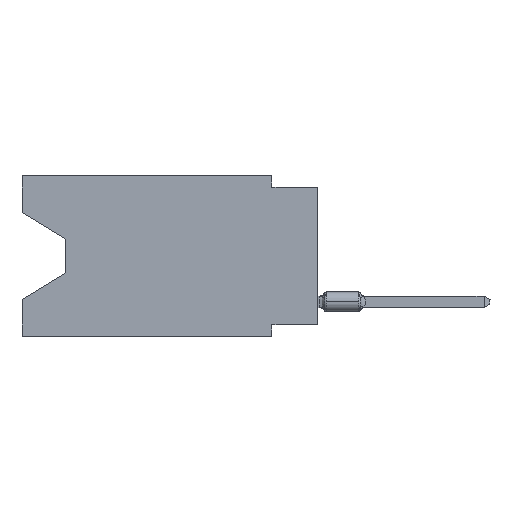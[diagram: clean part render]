
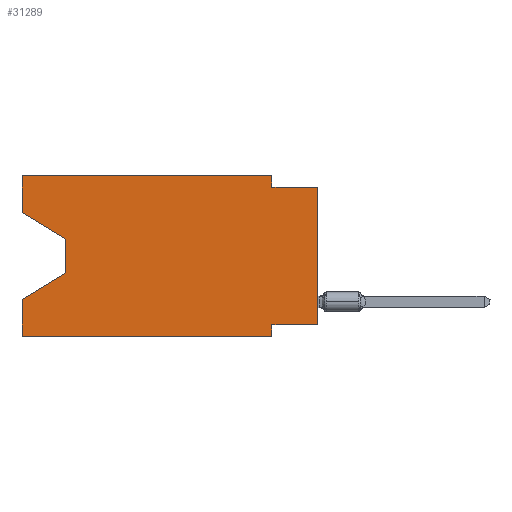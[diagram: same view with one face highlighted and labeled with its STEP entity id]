
A CAD part, left-side view. The second image highlights one B-rep face of the part: STEP entity #31289.
In plain terms, the highlighted planar face has unit normal (-1, 0, 0).
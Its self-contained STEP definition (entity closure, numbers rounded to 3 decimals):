
#288 = VERTEX_POINT ( 'NONE', #8696 ) ;
#362 = LINE ( 'NONE', #21409, #45308 ) ;
#1488 = CARTESIAN_POINT ( 'NONE',  ( 0., 13.97, -3.505 ) ) ;
#1493 = CARTESIAN_POINT ( 'NONE',  ( 0., 16.383, 0. ) ) ;
#2668 = VERTEX_POINT ( 'NONE', #25095 ) ;
#2764 = VECTOR ( 'NONE', #37496, 1000. ) ;
#3194 = ORIENTED_EDGE ( 'NONE', *, *, #24355, .F. ) ;
#3503 = ORIENTED_EDGE ( 'NONE', *, *, #11432, .T. ) ;
#3954 = VECTOR ( 'NONE', #22045, 1000. ) ;
#4253 = DIRECTION ( 'NONE',  ( 0., 1., 0. ) ) ;
#5149 = CARTESIAN_POINT ( 'NONE',  ( 0., 13.97, -5.385 ) ) ;
#5156 = EDGE_CURVE ( 'NONE', #2668, #15864, #10534, .T. ) ;
#5335 = CARTESIAN_POINT ( 'NONE',  ( 0., 16.383, -8.89 ) ) ;
#5417 = VERTEX_POINT ( 'NONE', #44933 ) ;
#5556 = VERTEX_POINT ( 'NONE', #24433 ) ;
#6807 = EDGE_CURVE ( 'NONE', #31838, #288, #43417, .T. ) ;
#7279 = CARTESIAN_POINT ( 'NONE',  ( 0., 16.383, 0. ) ) ;
#7749 = VECTOR ( 'NONE', #23061, 1000. ) ;
#8260 = CARTESIAN_POINT ( 'NONE',  ( 0., 16.383, -6.852 ) ) ;
#8550 = ORIENTED_EDGE ( 'NONE', *, *, #21426, .T. ) ;
#8588 = LINE ( 'NONE', #1493, #9632 ) ;
#8696 = CARTESIAN_POINT ( 'NONE',  ( 0., 2.54, -8.255 ) ) ;
#9279 = DIRECTION ( 'NONE',  ( 0., 0., -1. ) ) ;
#9632 = VECTOR ( 'NONE', #38292, 1000. ) ;
#9767 = VECTOR ( 'NONE', #20304, 1000. ) ;
#10534 = LINE ( 'NONE', #21626, #24575 ) ;
#11329 = LINE ( 'NONE', #5149, #2764 ) ;
#11432 = EDGE_CURVE ( 'NONE', #31838, #26762, #362, .T. ) ;
#11551 = DIRECTION ( 'NONE',  ( 0., 0., 1. ) ) ;
#12042 = ORIENTED_EDGE ( 'NONE', *, *, #6807, .F. ) ;
#13293 = VERTEX_POINT ( 'NONE', #8260 ) ;
#14489 = CARTESIAN_POINT ( 'NONE',  ( 0., 16.383, -2.038 ) ) ;
#15470 = EDGE_CURVE ( 'NONE', #21038, #5556, #22848, .T. ) ;
#15864 = VERTEX_POINT ( 'NONE', #22562 ) ;
#16681 = ORIENTED_EDGE ( 'NONE', *, *, #34973, .T. ) ;
#17640 = DIRECTION ( 'NONE',  ( 0., 0., -1. ) ) ;
#18025 = VECTOR ( 'NONE', #45277, 1000. ) ;
#18205 = EDGE_LOOP ( 'NONE', ( #16681, #8550, #35787, #31002, #39448, #19324, #12042, #3503, #3194, #38494, #41370, #25934 ) ) ;
#18444 = CARTESIAN_POINT ( 'NONE',  ( 0., 0., -8.255 ) ) ;
#18653 = EDGE_CURVE ( 'NONE', #22435, #13293, #11329, .T. ) ;
#19324 = ORIENTED_EDGE ( 'NONE', *, *, #32594, .F. ) ;
#19439 = VECTOR ( 'NONE', #9279, 1000. ) ;
#20145 = VECTOR ( 'NONE', #4253, 1000. ) ;
#20213 = VERTEX_POINT ( 'NONE', #24103 ) ;
#20304 = DIRECTION ( 'NONE',  ( 0., -1., 0. ) ) ;
#21038 = VERTEX_POINT ( 'NONE', #41430 ) ;
#21409 = CARTESIAN_POINT ( 'NONE',  ( 0., 0., 0. ) ) ;
#21426 = EDGE_CURVE ( 'NONE', #5417, #22435, #44442, .T. ) ;
#21626 = CARTESIAN_POINT ( 'NONE',  ( 0., 2.54, 0. ) ) ;
#22045 = DIRECTION ( 'NONE',  ( 0., -1., 0. ) ) ;
#22176 = CARTESIAN_POINT ( 'NONE',  ( 0., 16.383, 0. ) ) ;
#22183 = FACE_OUTER_BOUND ( 'NONE', #18205, .T. ) ;
#22435 = VERTEX_POINT ( 'NONE', #28856 ) ;
#22562 = CARTESIAN_POINT ( 'NONE',  ( 0., 2.54, -0.635 ) ) ;
#22848 = LINE ( 'NONE', #5335, #7749 ) ;
#23061 = DIRECTION ( 'NONE',  ( 0., -1., 0. ) ) ;
#24103 = CARTESIAN_POINT ( 'NONE',  ( 0., 16.383, 0. ) ) ;
#24355 = EDGE_CURVE ( 'NONE', #15864, #26762, #34714, .T. ) ;
#24433 = CARTESIAN_POINT ( 'NONE',  ( 0., 2.54, -8.89 ) ) ;
#24575 = VECTOR ( 'NONE', #17640, 1000. ) ;
#25095 = CARTESIAN_POINT ( 'NONE',  ( 0., 2.54, 0. ) ) ;
#25823 = LINE ( 'NONE', #14489, #29602 ) ;
#25934 = ORIENTED_EDGE ( 'NONE', *, *, #32847, .F. ) ;
#26762 = VERTEX_POINT ( 'NONE', #33338 ) ;
#27615 = CARTESIAN_POINT ( 'NONE',  ( 0., 0., -0.635 ) ) ;
#28650 = LINE ( 'NONE', #46530, #3954 ) ;
#28856 = CARTESIAN_POINT ( 'NONE',  ( 0., 13.97, -5.385 ) ) ;
#29028 = DIRECTION ( 'NONE',  ( 0., 0., -1. ) ) ;
#29450 = CARTESIAN_POINT ( 'NONE',  ( 0., 0., -8.255 ) ) ;
#29602 = VECTOR ( 'NONE', #36197, 1000. ) ;
#31002 = ORIENTED_EDGE ( 'NONE', *, *, #45710, .F. ) ;
#31151 = LINE ( 'NONE', #37999, #18025 ) ;
#31289 = ADVANCED_FACE ( 'NONE', ( #22183 ), #35637, .F. ) ;
#31726 = VECTOR ( 'NONE', #11551, 1000. ) ;
#31838 = VERTEX_POINT ( 'NONE', #29450 ) ;
#32594 = EDGE_CURVE ( 'NONE', #288, #5556, #31151, .T. ) ;
#32847 = EDGE_CURVE ( 'NONE', #44075, #20213, #33507, .T. ) ;
#33338 = CARTESIAN_POINT ( 'NONE',  ( 0., 0., -0.635 ) ) ;
#33507 = LINE ( 'NONE', #22176, #31726 ) ;
#34714 = LINE ( 'NONE', #27615, #9767 ) ;
#34959 = EDGE_CURVE ( 'NONE', #20213, #2668, #28650, .T. ) ;
#34973 = EDGE_CURVE ( 'NONE', #44075, #5417, #25823, .T. ) ;
#35637 = PLANE ( 'NONE',  #44527 ) ;
#35787 = ORIENTED_EDGE ( 'NONE', *, *, #18653, .T. ) ;
#36197 = DIRECTION ( 'NONE',  ( 0., -0.855, -0.519 ) ) ;
#37496 = DIRECTION ( 'NONE',  ( 0., 0.855, -0.519 ) ) ;
#37999 = CARTESIAN_POINT ( 'NONE',  ( 0., 2.54, -8.89 ) ) ;
#38292 = DIRECTION ( 'NONE',  ( 0., 0., 1. ) ) ;
#38494 = ORIENTED_EDGE ( 'NONE', *, *, #5156, .F. ) ;
#39448 = ORIENTED_EDGE ( 'NONE', *, *, #15470, .T. ) ;
#41370 = ORIENTED_EDGE ( 'NONE', *, *, #34959, .F. ) ;
#41430 = CARTESIAN_POINT ( 'NONE',  ( 0., 16.383, -8.89 ) ) ;
#43383 = DIRECTION ( 'NONE',  ( 1., 0., 0. ) ) ;
#43417 = LINE ( 'NONE', #18444, #20145 ) ;
#44075 = VERTEX_POINT ( 'NONE', #44729 ) ;
#44442 = LINE ( 'NONE', #1488, #19439 ) ;
#44527 = AXIS2_PLACEMENT_3D ( 'NONE', #7279, #43383, #29028 ) ;
#44729 = CARTESIAN_POINT ( 'NONE',  ( 0., 16.383, -2.038 ) ) ;
#44933 = CARTESIAN_POINT ( 'NONE',  ( 0., 13.97, -3.505 ) ) ;
#45277 = DIRECTION ( 'NONE',  ( 0., 0., -1. ) ) ;
#45308 = VECTOR ( 'NONE', #46152, 1000. ) ;
#45710 = EDGE_CURVE ( 'NONE', #21038, #13293, #8588, .T. ) ;
#46152 = DIRECTION ( 'NONE',  ( 0., 0., 1. ) ) ;
#46530 = CARTESIAN_POINT ( 'NONE',  ( 0., 16.383, 0. ) ) ;
